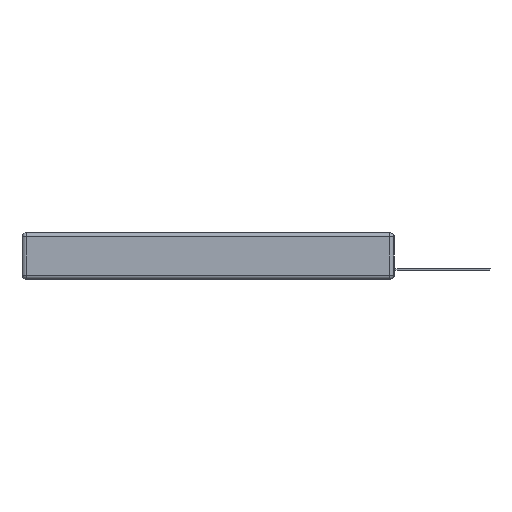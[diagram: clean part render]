
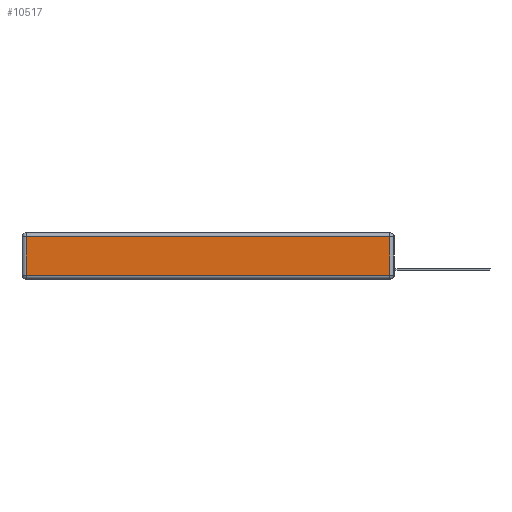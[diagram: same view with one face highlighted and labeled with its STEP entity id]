
A CAD part, left-side view. The second image highlights one B-rep face of the part: STEP entity #10517.
In plain terms, the highlighted planar face has unit normal (-1, 0, 0).
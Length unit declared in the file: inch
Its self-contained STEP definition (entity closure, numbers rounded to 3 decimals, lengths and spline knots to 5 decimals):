
#999 = DIRECTION ( 'NONE',  ( 0., 0., 1. ) ) ;
#1087 = VERTEX_POINT ( 'NONE', #3828 ) ;
#2007 = DIRECTION ( 'NONE',  ( 0., 0., 1. ) ) ;
#2281 = VECTOR ( 'NONE', #9139, 39.37008 ) ;
#3194 = CARTESIAN_POINT ( 'NONE',  ( 0., 0.03, -0.03 ) ) ;
#3220 = PLANE ( 'NONE',  #10921 ) ;
#3428 = EDGE_CURVE ( 'NONE', #1087, #12685, #14460, .T. ) ;
#3452 = VERTEX_POINT ( 'NONE', #9576 ) ;
#3594 = VECTOR ( 'NONE', #12134, 39.37008 ) ;
#3828 = CARTESIAN_POINT ( 'NONE',  ( 0., 0.03, -0.313 ) ) ;
#4016 = VECTOR ( 'NONE', #10227, 39.37008 ) ;
#5397 = EDGE_CURVE ( 'NONE', #12685, #5476, #8610, .T. ) ;
#5476 = VERTEX_POINT ( 'NONE', #13823 ) ;
#5577 = CARTESIAN_POINT ( 'NONE',  ( 0., 0., -0.313 ) ) ;
#7645 = DIRECTION ( 'NONE',  ( -1., 0., 0. ) ) ;
#7802 = ORIENTED_EDGE ( 'NONE', *, *, #11630, .T. ) ;
#8610 = LINE ( 'NONE', #14382, #2281 ) ;
#8625 = EDGE_CURVE ( 'NONE', #5476, #3452, #11831, .T. ) ;
#9139 = DIRECTION ( 'NONE',  ( 0., 1., 0. ) ) ;
#9554 = VECTOR ( 'NONE', #2007, 39.37008 ) ;
#9576 = CARTESIAN_POINT ( 'NONE',  ( 0., 2.72, -0.313 ) ) ;
#10227 = DIRECTION ( 'NONE',  ( 0., -1., 0. ) ) ;
#10517 = ADVANCED_FACE ( 'NONE', ( #10533 ), #3220, .T. ) ;
#10533 = FACE_OUTER_BOUND ( 'NONE', #10712, .T. ) ;
#10712 = EDGE_LOOP ( 'NONE', ( #7802, #13408, #13420, #11758 ) ) ;
#10921 = AXIS2_PLACEMENT_3D ( 'NONE', #14344, #7645, #999 ) ;
#11066 = CARTESIAN_POINT ( 'NONE',  ( 0., 2.72, -0.343 ) ) ;
#11552 = LINE ( 'NONE', #5577, #4016 ) ;
#11630 = EDGE_CURVE ( 'NONE', #3452, #1087, #11552, .T. ) ;
#11758 = ORIENTED_EDGE ( 'NONE', *, *, #8625, .T. ) ;
#11831 = LINE ( 'NONE', #11066, #3594 ) ;
#12121 = CARTESIAN_POINT ( 'NONE',  ( 0., 0.03, -0.343 ) ) ;
#12134 = DIRECTION ( 'NONE',  ( 0., 0., -1. ) ) ;
#12685 = VERTEX_POINT ( 'NONE', #3194 ) ;
#13408 = ORIENTED_EDGE ( 'NONE', *, *, #3428, .T. ) ;
#13420 = ORIENTED_EDGE ( 'NONE', *, *, #5397, .T. ) ;
#13823 = CARTESIAN_POINT ( 'NONE',  ( 0., 2.72, -0.03 ) ) ;
#14344 = CARTESIAN_POINT ( 'NONE',  ( 0., 0., -0.343 ) ) ;
#14382 = CARTESIAN_POINT ( 'NONE',  ( 0., 2.75, -0.03 ) ) ;
#14460 = LINE ( 'NONE', #12121, #9554 ) ;
